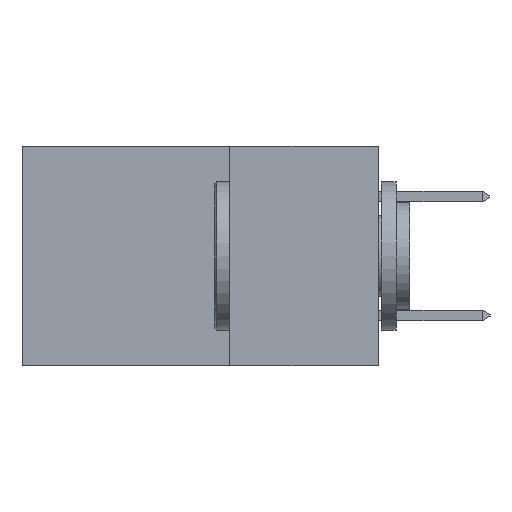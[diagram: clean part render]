
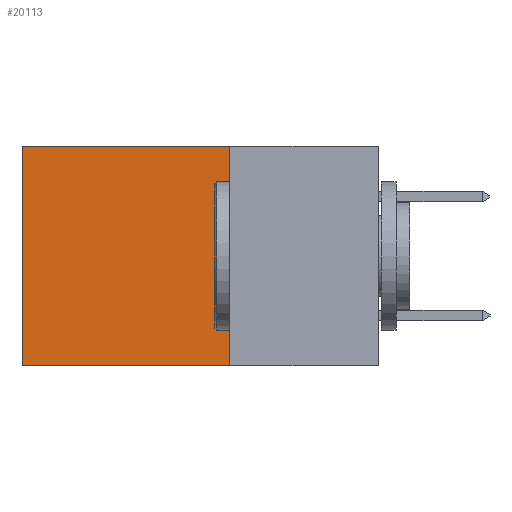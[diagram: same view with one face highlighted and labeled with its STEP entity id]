
A CAD part, left-side view. The second image highlights one B-rep face of the part: STEP entity #20113.
In plain terms, the highlighted planar face has unit normal (-1, 0, 0).
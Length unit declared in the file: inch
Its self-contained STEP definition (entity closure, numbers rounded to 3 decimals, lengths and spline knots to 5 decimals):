
#188 = DIRECTION ( 'NONE',  ( 0., 1., 0. ) ) ;
#275 = CARTESIAN_POINT ( 'NONE',  ( 0.2615, 0.25, 0. ) ) ;
#311 = EDGE_LOOP ( 'NONE', ( #15683, #5435, #4197, #6068 ) ) ;
#673 = CARTESIAN_POINT ( 'NONE',  ( 0.2615, 0.25, -0.37 ) ) ;
#1709 = CARTESIAN_POINT ( 'NONE',  ( 0.2615, 0.6, -0.37 ) ) ;
#2248 = VERTEX_POINT ( 'NONE', #20186 ) ;
#4197 = ORIENTED_EDGE ( 'NONE', *, *, #9244, .F. ) ;
#4306 = LINE ( 'NONE', #5130, #10088 ) ;
#4665 = EDGE_CURVE ( 'NONE', #2248, #13562, #9093, .T. ) ;
#5081 = EDGE_CURVE ( 'NONE', #18196, #12136, #20110, .T. ) ;
#5130 = CARTESIAN_POINT ( 'NONE',  ( 0.2615, 0.25, -0.37 ) ) ;
#5435 = ORIENTED_EDGE ( 'NONE', *, *, #5081, .F. ) ;
#6068 = ORIENTED_EDGE ( 'NONE', *, *, #4665, .T. ) ;
#9093 = LINE ( 'NONE', #275, #19510 ) ;
#9244 = EDGE_CURVE ( 'NONE', #2248, #18196, #4306, .T. ) ;
#9844 = CARTESIAN_POINT ( 'NONE',  ( 0.2615, 0.6, -0.37 ) ) ;
#10088 = VECTOR ( 'NONE', #18792, 39.37008 ) ;
#10974 = DIRECTION ( 'NONE',  ( 1., 0., 0. ) ) ;
#11019 = VECTOR ( 'NONE', #13779, 39.37008 ) ;
#12136 = VERTEX_POINT ( 'NONE', #1709 ) ;
#13562 = VERTEX_POINT ( 'NONE', #15223 ) ;
#13779 = DIRECTION ( 'NONE',  ( 0., 0., -1. ) ) ;
#15223 = CARTESIAN_POINT ( 'NONE',  ( 0.2615, 0.6, 0. ) ) ;
#15683 = ORIENTED_EDGE ( 'NONE', *, *, #25149, .T. ) ;
#15685 = AXIS2_PLACEMENT_3D ( 'NONE', #18791, #10974, #24659 ) ;
#16253 = LINE ( 'NONE', #9844, #11019 ) ;
#16284 = FACE_OUTER_BOUND ( 'NONE', #311, .T. ) ;
#18196 = VERTEX_POINT ( 'NONE', #673 ) ;
#18791 = CARTESIAN_POINT ( 'NONE',  ( 0.2615, 0.25, -0.37 ) ) ;
#18792 = DIRECTION ( 'NONE',  ( 0., 0., -1. ) ) ;
#19489 = VECTOR ( 'NONE', #20740, 39.37008 ) ;
#19510 = VECTOR ( 'NONE', #188, 39.37008 ) ;
#20110 = LINE ( 'NONE', #20877, #19489 ) ;
#20113 = ADVANCED_FACE ( 'NONE', ( #16284 ), #22678, .F. ) ;
#20186 = CARTESIAN_POINT ( 'NONE',  ( 0.2615, 0.25, 0. ) ) ;
#20740 = DIRECTION ( 'NONE',  ( 0., 1., 0. ) ) ;
#20877 = CARTESIAN_POINT ( 'NONE',  ( 0.2615, 0.25, -0.37 ) ) ;
#22678 = PLANE ( 'NONE',  #15685 ) ;
#24659 = DIRECTION ( 'NONE',  ( 0., 0., -1. ) ) ;
#25149 = EDGE_CURVE ( 'NONE', #13562, #12136, #16253, .T. ) ;
